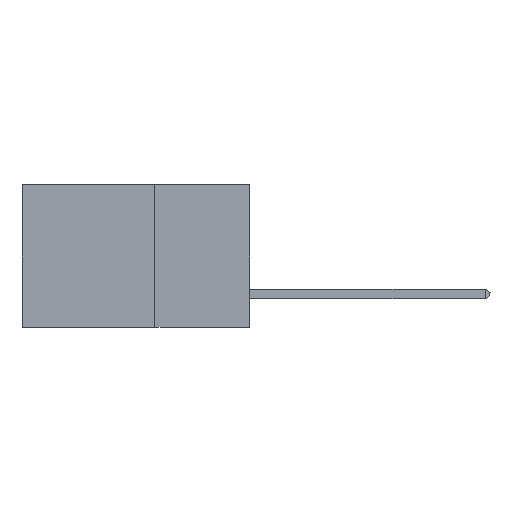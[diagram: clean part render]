
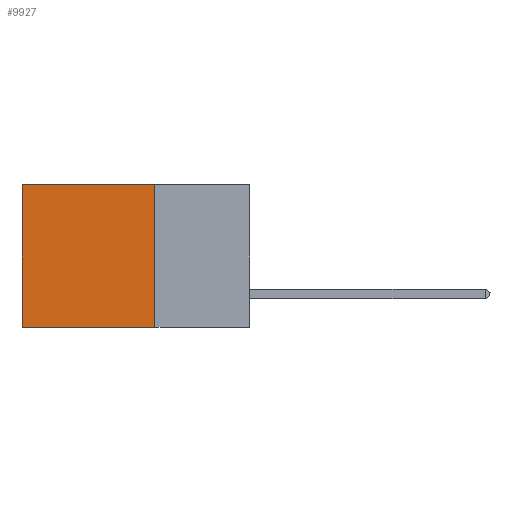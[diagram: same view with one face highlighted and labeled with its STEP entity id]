
A CAD part, left-side view. The second image highlights one B-rep face of the part: STEP entity #9927.
In plain terms, the highlighted planar face has unit normal (-1, 0, 0).
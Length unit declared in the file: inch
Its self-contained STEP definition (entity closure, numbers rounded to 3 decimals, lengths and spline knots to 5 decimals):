
#799 = PLANE ( 'NONE',  #7671 ) ;
#1870 = VERTEX_POINT ( 'NONE', #13003 ) ;
#2071 = LINE ( 'NONE', #9167, #7379 ) ;
#2322 = CARTESIAN_POINT ( 'NONE',  ( 0.2875, 0.25, -0.375 ) ) ;
#2603 = VECTOR ( 'NONE', #3312, 39.37008 ) ;
#2619 = EDGE_CURVE ( 'NONE', #6183, #1870, #3501, .T. ) ;
#2805 = CARTESIAN_POINT ( 'NONE',  ( 0.2875, 0.25, -0.375 ) ) ;
#3312 = DIRECTION ( 'NONE',  ( 0., 1., 0. ) ) ;
#3416 = VECTOR ( 'NONE', #10005, 39.37008 ) ;
#3501 = LINE ( 'NONE', #4440, #2603 ) ;
#3801 = DIRECTION ( 'NONE',  ( 0., 1., 0. ) ) ;
#4440 = CARTESIAN_POINT ( 'NONE',  ( 0.2875, 0.25, 0. ) ) ;
#5100 = EDGE_CURVE ( 'NONE', #9531, #12836, #12872, .T. ) ;
#5867 = ORIENTED_EDGE ( 'NONE', *, *, #6129, .F. ) ;
#6129 = EDGE_CURVE ( 'NONE', #6183, #9531, #2071, .T. ) ;
#6183 = VERTEX_POINT ( 'NONE', #11615 ) ;
#6210 = DIRECTION ( 'NONE',  ( 0., 0., -1. ) ) ;
#6241 = VECTOR ( 'NONE', #3801, 39.37008 ) ;
#6850 = ORIENTED_EDGE ( 'NONE', *, *, #10545, .T. ) ;
#7201 = LINE ( 'NONE', #11277, #3416 ) ;
#7379 = VECTOR ( 'NONE', #6210, 39.37008 ) ;
#7570 = EDGE_LOOP ( 'NONE', ( #6850, #11347, #5867, #9411 ) ) ;
#7671 = AXIS2_PLACEMENT_3D ( 'NONE', #7957, #8951, #12335 ) ;
#7957 = CARTESIAN_POINT ( 'NONE',  ( 0.2875, 0.25, -0.375 ) ) ;
#8361 = CARTESIAN_POINT ( 'NONE',  ( 0.2875, 0.6, -0.375 ) ) ;
#8951 = DIRECTION ( 'NONE',  ( 1., 0., 0. ) ) ;
#9167 = CARTESIAN_POINT ( 'NONE',  ( 0.2875, 0.25, -0.375 ) ) ;
#9411 = ORIENTED_EDGE ( 'NONE', *, *, #2619, .T. ) ;
#9531 = VERTEX_POINT ( 'NONE', #2322 ) ;
#9927 = ADVANCED_FACE ( 'NONE', ( #9940 ), #799, .F. ) ;
#9940 = FACE_OUTER_BOUND ( 'NONE', #7570, .T. ) ;
#10005 = DIRECTION ( 'NONE',  ( 0., 0., -1. ) ) ;
#10545 = EDGE_CURVE ( 'NONE', #1870, #12836, #7201, .T. ) ;
#11277 = CARTESIAN_POINT ( 'NONE',  ( 0.2875, 0.6, -0.375 ) ) ;
#11347 = ORIENTED_EDGE ( 'NONE', *, *, #5100, .F. ) ;
#11615 = CARTESIAN_POINT ( 'NONE',  ( 0.2875, 0.25, 0. ) ) ;
#12335 = DIRECTION ( 'NONE',  ( 0., 0., -1. ) ) ;
#12836 = VERTEX_POINT ( 'NONE', #8361 ) ;
#12872 = LINE ( 'NONE', #2805, #6241 ) ;
#13003 = CARTESIAN_POINT ( 'NONE',  ( 0.2875, 0.6, 0. ) ) ;
